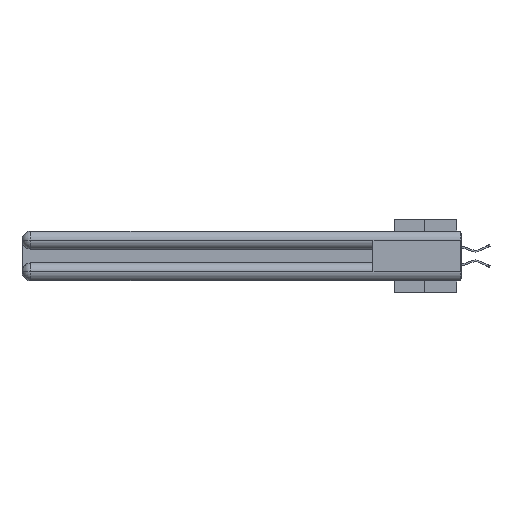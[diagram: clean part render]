
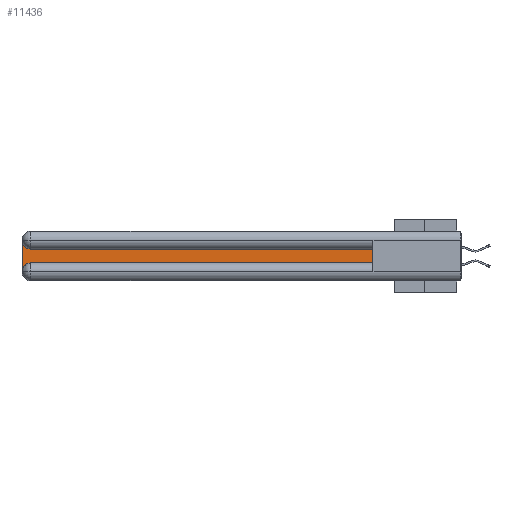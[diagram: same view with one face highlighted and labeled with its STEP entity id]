
A CAD part, left-side view. The second image highlights one B-rep face of the part: STEP entity #11436.
In plain terms, the highlighted planar face has unit normal (-1, 0, 0).
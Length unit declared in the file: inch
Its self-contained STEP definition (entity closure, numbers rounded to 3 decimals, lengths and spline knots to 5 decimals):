
#3998 = ORIENTED_EDGE ( 'NONE', *, *, #24264, .T. ) ;
#4527 = VERTEX_POINT ( 'NONE', #31178 ) ;
#4855 = VECTOR ( 'NONE', #26900, 39.37008 ) ;
#5406 = DIRECTION ( 'NONE',  ( 1., 0., 0. ) ) ;
#6284 = EDGE_CURVE ( 'NONE', #10917, #35276, #6554, .T. ) ;
#6554 = LINE ( 'NONE', #37920, #14079 ) ;
#8067 = CARTESIAN_POINT ( 'NONE',  ( 0.075, 2.94, -0.2775 ) ) ;
#9793 = EDGE_CURVE ( 'NONE', #4527, #10917, #25879, .T. ) ;
#10027 = ORIENTED_EDGE ( 'NONE', *, *, #13833, .T. ) ;
#10917 = VERTEX_POINT ( 'NONE', #34834 ) ;
#10974 = VERTEX_POINT ( 'NONE', #25287 ) ;
#11080 = EDGE_CURVE ( 'NONE', #24323, #4527, #23283, .T. ) ;
#11333 = CARTESIAN_POINT ( 'NONE',  ( 0.075, 0.6, -0.1225 ) ) ;
#11436 = ADVANCED_FACE ( 'NONE', ( #25224 ), #21651, .F. ) ;
#13263 = CARTESIAN_POINT ( 'NONE',  ( 0.075, 3., -0.2775 ) ) ;
#13422 = LINE ( 'NONE', #39324, #4855 ) ;
#13833 = EDGE_CURVE ( 'NONE', #10974, #38165, #13422, .T. ) ;
#14079 = VECTOR ( 'NONE', #31571, 39.37008 ) ;
#14783 = CARTESIAN_POINT ( 'NONE',  ( 0.075, 0.6, -0.2175 ) ) ;
#15092 = DIRECTION ( 'NONE',  ( 1., 0., 0. ) ) ;
#15496 = DIRECTION ( 'NONE',  ( 0., 0., -1. ) ) ;
#19143 = DIRECTION ( 'NONE',  ( 1., 0., 0. ) ) ;
#19254 = DIRECTION ( 'NONE',  ( 0., 1., 0. ) ) ;
#19556 = LINE ( 'NONE', #37193, #31587 ) ;
#21651 = PLANE ( 'NONE',  #32911 ) ;
#23283 = LINE ( 'NONE', #31895, #31288 ) ;
#24264 = EDGE_CURVE ( 'NONE', #38165, #24323, #19556, .T. ) ;
#24323 = VERTEX_POINT ( 'NONE', #11333 ) ;
#24558 = ORIENTED_EDGE ( 'NONE', *, *, #9793, .T. ) ;
#25224 = FACE_OUTER_BOUND ( 'NONE', #40682, .T. ) ;
#25287 = CARTESIAN_POINT ( 'NONE',  ( 0.075, 2.94, -0.2175 ) ) ;
#25879 = CIRCLE ( 'NONE', #39334, 0.06 ) ;
#26593 = ORIENTED_EDGE ( 'NONE', *, *, #6284, .T. ) ;
#26900 = DIRECTION ( 'NONE',  ( 0., -1., 0. ) ) ;
#27125 = ORIENTED_EDGE ( 'NONE', *, *, #34863, .T. ) ;
#28695 = CARTESIAN_POINT ( 'NONE',  ( 0.075, 2.94, -0.0625 ) ) ;
#30486 = AXIS2_PLACEMENT_3D ( 'NONE', #8067, #5406, #31094 ) ;
#31094 = DIRECTION ( 'NONE',  ( 0., 0., -1. ) ) ;
#31178 = CARTESIAN_POINT ( 'NONE',  ( 0.075, 2.94, -0.1225 ) ) ;
#31288 = VECTOR ( 'NONE', #19254, 39.37008 ) ;
#31299 = CIRCLE ( 'NONE', #30486, 0.06 ) ;
#31367 = CARTESIAN_POINT ( 'NONE',  ( 0.075, 3., -0.1225 ) ) ;
#31571 = DIRECTION ( 'NONE',  ( 0., 0., -1. ) ) ;
#31587 = VECTOR ( 'NONE', #40435, 39.37008 ) ;
#31895 = CARTESIAN_POINT ( 'NONE',  ( 0.075, 0.6, -0.1225 ) ) ;
#32911 = AXIS2_PLACEMENT_3D ( 'NONE', #31367, #15092, #37724 ) ;
#34834 = CARTESIAN_POINT ( 'NONE',  ( 0.075, 3., -0.0625 ) ) ;
#34863 = EDGE_CURVE ( 'NONE', #35276, #10974, #31299, .T. ) ;
#35276 = VERTEX_POINT ( 'NONE', #13263 ) ;
#37193 = CARTESIAN_POINT ( 'NONE',  ( 0.075, 0.6, -0.2175 ) ) ;
#37724 = DIRECTION ( 'NONE',  ( 0., 0., -1. ) ) ;
#37920 = CARTESIAN_POINT ( 'NONE',  ( 0.075, 3., -0.2175 ) ) ;
#38165 = VERTEX_POINT ( 'NONE', #14783 ) ;
#38186 = ORIENTED_EDGE ( 'NONE', *, *, #11080, .T. ) ;
#39324 = CARTESIAN_POINT ( 'NONE',  ( 0.075, 0.6, -0.2175 ) ) ;
#39334 = AXIS2_PLACEMENT_3D ( 'NONE', #28695, #19143, #15496 ) ;
#40435 = DIRECTION ( 'NONE',  ( 0., 0., 1. ) ) ;
#40682 = EDGE_LOOP ( 'NONE', ( #38186, #24558, #26593, #27125, #10027, #3998 ) ) ;
